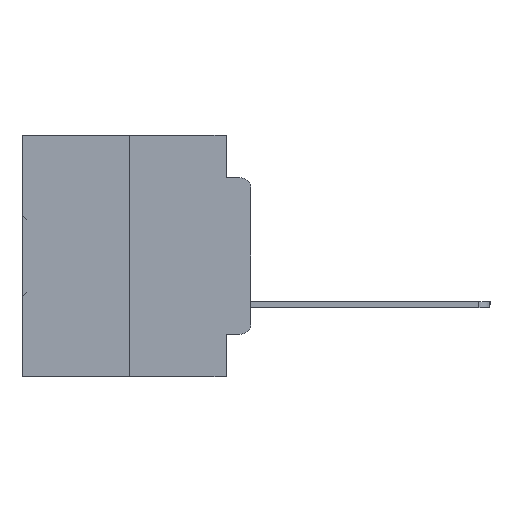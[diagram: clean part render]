
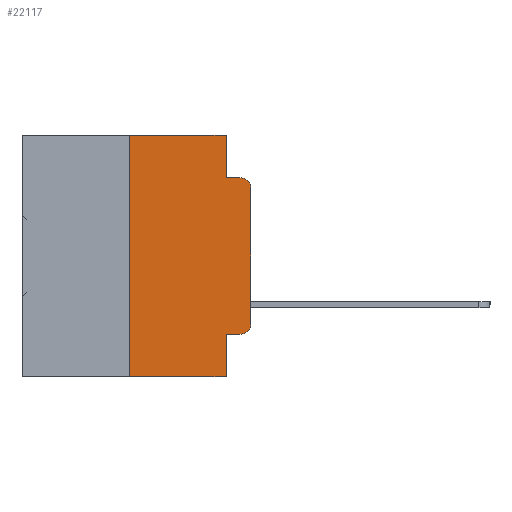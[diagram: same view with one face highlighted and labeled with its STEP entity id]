
A CAD part, left-side view. The second image highlights one B-rep face of the part: STEP entity #22117.
In plain terms, the highlighted planar face has unit normal (-1, 0, 0).
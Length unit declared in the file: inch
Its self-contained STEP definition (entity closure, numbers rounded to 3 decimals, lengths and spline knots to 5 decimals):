
#10 = DIRECTION ( 'NONE',  ( 0., 0., -1. ) ) ;
#365 = EDGE_LOOP ( 'NONE', ( #9604, #25569, #29003, #12784, #34901, #20268, #12284, #25534, #3631, #27058 ) ) ;
#636 = CARTESIAN_POINT ( 'NONE',  ( 0., 0.25, 0. ) ) ;
#990 = VECTOR ( 'NONE', #16092, 39.37008 ) ;
#3631 = ORIENTED_EDGE ( 'NONE', *, *, #36657, .T. ) ;
#5134 = VERTEX_POINT ( 'NONE', #26378 ) ;
#5594 = CARTESIAN_POINT ( 'NONE',  ( 0., 0.051, -0.4115 ) ) ;
#5687 = FACE_OUTER_BOUND ( 'NONE', #365, .T. ) ;
#5871 = CARTESIAN_POINT ( 'NONE',  ( 0., 0.473, 0. ) ) ;
#5980 = VECTOR ( 'NONE', #11102, 39.37008 ) ;
#6520 = VERTEX_POINT ( 'NONE', #636 ) ;
#7745 = EDGE_CURVE ( 'NONE', #26137, #19492, #14856, .T. ) ;
#9604 = ORIENTED_EDGE ( 'NONE', *, *, #19829, .T. ) ;
#9718 = LINE ( 'NONE', #23437, #31514 ) ;
#10101 = CARTESIAN_POINT ( 'NONE',  ( 0., 0.051, 0. ) ) ;
#11102 = DIRECTION ( 'NONE',  ( 0., -1., 0. ) ) ;
#11145 = DIRECTION ( 'NONE',  ( 1., 0., 0. ) ) ;
#12284 = ORIENTED_EDGE ( 'NONE', *, *, #22538, .T. ) ;
#12449 = VECTOR ( 'NONE', #19236, 39.37008 ) ;
#12784 = ORIENTED_EDGE ( 'NONE', *, *, #7745, .F. ) ;
#12938 = LINE ( 'NONE', #31942, #13735 ) ;
#13552 = EDGE_CURVE ( 'NONE', #13623, #21494, #29644, .T. ) ;
#13623 = VERTEX_POINT ( 'NONE', #26061 ) ;
#13735 = VECTOR ( 'NONE', #29137, 39.37008 ) ;
#14569 = CARTESIAN_POINT ( 'NONE',  ( 0., 0.02, -0.1085 ) ) ;
#14656 = EDGE_CURVE ( 'NONE', #18426, #6520, #33969, .T. ) ;
#14755 = DIRECTION ( 'NONE',  ( 0., 0., -1. ) ) ;
#14806 = VERTEX_POINT ( 'NONE', #17065 ) ;
#14840 = CIRCLE ( 'NONE', #35822, 0.02 ) ;
#14856 = LINE ( 'NONE', #17861, #19326 ) ;
#15011 = EDGE_CURVE ( 'NONE', #19492, #5134, #9718, .T. ) ;
#15204 = CARTESIAN_POINT ( 'NONE',  ( 0., 0., -0.1085 ) ) ;
#16092 = DIRECTION ( 'NONE',  ( 0., 0., -1. ) ) ;
#16881 = CARTESIAN_POINT ( 'NONE',  ( 0., 0.25, 0. ) ) ;
#17065 = CARTESIAN_POINT ( 'NONE',  ( 0., 0.051, -0.5 ) ) ;
#17232 = VECTOR ( 'NONE', #36945, 39.37008 ) ;
#17429 = DIRECTION ( 'NONE',  ( 0., 0., -1. ) ) ;
#17675 = EDGE_CURVE ( 'NONE', #32681, #14806, #21930, .T. ) ;
#17861 = CARTESIAN_POINT ( 'NONE',  ( 0., 0.051, 0. ) ) ;
#18121 = EDGE_CURVE ( 'NONE', #6520, #26137, #30690, .T. ) ;
#18315 = VECTOR ( 'NONE', #28154, 39.37008 ) ;
#18426 = VERTEX_POINT ( 'NONE', #31980 ) ;
#18584 = AXIS2_PLACEMENT_3D ( 'NONE', #5871, #11145, #10 ) ;
#19236 = DIRECTION ( 'NONE',  ( 0., -1., 0. ) ) ;
#19326 = VECTOR ( 'NONE', #34948, 39.37008 ) ;
#19492 = VERTEX_POINT ( 'NONE', #26912 ) ;
#19829 = EDGE_CURVE ( 'NONE', #21494, #26816, #12938, .T. ) ;
#19953 = CARTESIAN_POINT ( 'NONE',  ( 0., 0.051, 0. ) ) ;
#20268 = ORIENTED_EDGE ( 'NONE', *, *, #14656, .F. ) ;
#21494 = VERTEX_POINT ( 'NONE', #28736 ) ;
#21930 = LINE ( 'NONE', #10101, #990 ) ;
#22117 = ADVANCED_FACE ( 'NONE', ( #5687 ), #31580, .F. ) ;
#22538 = EDGE_CURVE ( 'NONE', #18426, #14806, #22566, .T. ) ;
#22566 = LINE ( 'NONE', #36818, #5980 ) ;
#23219 = DIRECTION ( 'NONE',  ( -1., 0., 0. ) ) ;
#23437 = CARTESIAN_POINT ( 'NONE',  ( 0., 0.051, -0.0885 ) ) ;
#24699 = CARTESIAN_POINT ( 'NONE',  ( 0., 0.473, 0. ) ) ;
#25511 = DIRECTION ( 'NONE',  ( -1., 0., 0. ) ) ;
#25534 = ORIENTED_EDGE ( 'NONE', *, *, #17675, .F. ) ;
#25569 = ORIENTED_EDGE ( 'NONE', *, *, #33314, .T. ) ;
#26061 = CARTESIAN_POINT ( 'NONE',  ( 0., 0.02, -0.4115 ) ) ;
#26137 = VERTEX_POINT ( 'NONE', #19953 ) ;
#26378 = CARTESIAN_POINT ( 'NONE',  ( 0., 0.02, -0.0885 ) ) ;
#26816 = VERTEX_POINT ( 'NONE', #15204 ) ;
#26912 = CARTESIAN_POINT ( 'NONE',  ( 0., 0.051, -0.0885 ) ) ;
#27058 = ORIENTED_EDGE ( 'NONE', *, *, #13552, .T. ) ;
#28154 = DIRECTION ( 'NONE',  ( 0., 0., 1. ) ) ;
#28736 = CARTESIAN_POINT ( 'NONE',  ( 0., 0., -0.3915 ) ) ;
#29003 = ORIENTED_EDGE ( 'NONE', *, *, #15011, .F. ) ;
#29137 = DIRECTION ( 'NONE',  ( 0., 0., 1. ) ) ;
#29644 = CIRCLE ( 'NONE', #36861, 0.02 ) ;
#30690 = LINE ( 'NONE', #24699, #12449 ) ;
#31313 = LINE ( 'NONE', #5594, #17232 ) ;
#31514 = VECTOR ( 'NONE', #34691, 39.37008 ) ;
#31580 = PLANE ( 'NONE',  #18584 ) ;
#31878 = CARTESIAN_POINT ( 'NONE',  ( 0., 0.02, -0.3915 ) ) ;
#31942 = CARTESIAN_POINT ( 'NONE',  ( 0., 0., 0. ) ) ;
#31980 = CARTESIAN_POINT ( 'NONE',  ( 0., 0.25, -0.5 ) ) ;
#32681 = VERTEX_POINT ( 'NONE', #33639 ) ;
#33314 = EDGE_CURVE ( 'NONE', #26816, #5134, #14840, .T. ) ;
#33639 = CARTESIAN_POINT ( 'NONE',  ( 0., 0.051, -0.4115 ) ) ;
#33969 = LINE ( 'NONE', #16881, #18315 ) ;
#34691 = DIRECTION ( 'NONE',  ( 0., -1., 0. ) ) ;
#34901 = ORIENTED_EDGE ( 'NONE', *, *, #18121, .F. ) ;
#34948 = DIRECTION ( 'NONE',  ( 0., 0., -1. ) ) ;
#35822 = AXIS2_PLACEMENT_3D ( 'NONE', #14569, #23219, #14755 ) ;
#36657 = EDGE_CURVE ( 'NONE', #32681, #13623, #31313, .T. ) ;
#36818 = CARTESIAN_POINT ( 'NONE',  ( 0., 0.473, -0.5 ) ) ;
#36861 = AXIS2_PLACEMENT_3D ( 'NONE', #31878, #25511, #17429 ) ;
#36945 = DIRECTION ( 'NONE',  ( 0., -1., 0. ) ) ;
